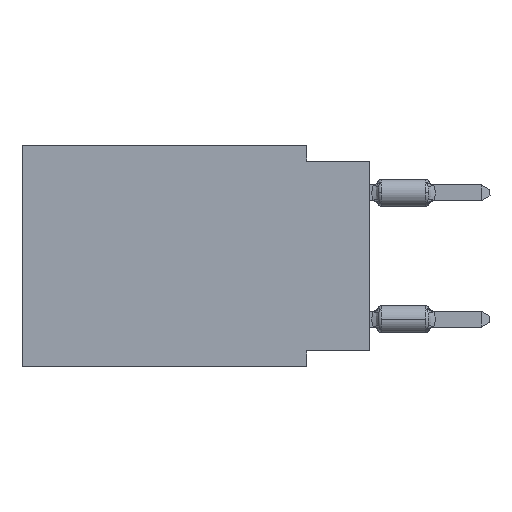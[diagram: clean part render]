
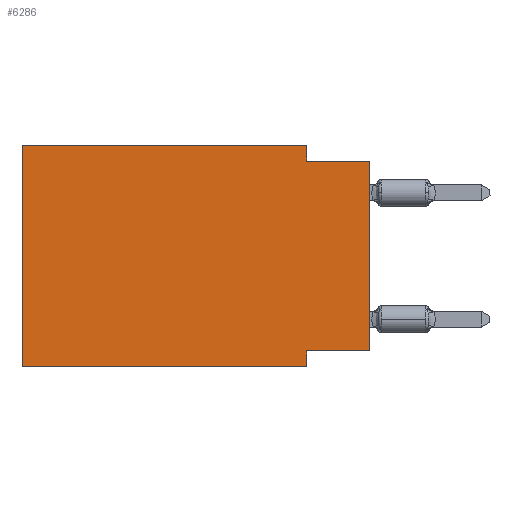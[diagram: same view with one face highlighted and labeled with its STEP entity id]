
A CAD part, left-side view. The second image highlights one B-rep face of the part: STEP entity #6286.
In plain terms, the highlighted planar face has unit normal (-1, 0, 0).
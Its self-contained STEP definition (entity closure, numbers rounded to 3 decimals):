
#235 = CARTESIAN_POINT ( 'NONE',  ( 0., 13.97, 0. ) ) ;
#1528 = LINE ( 'NONE', #235, #7803 ) ;
#1599 = ORIENTED_EDGE ( 'NONE', *, *, #19252, .T. ) ;
#1711 = ORIENTED_EDGE ( 'NONE', *, *, #14318, .F. ) ;
#1934 = LINE ( 'NONE', #18508, #4574 ) ;
#2109 = EDGE_CURVE ( 'NONE', #11399, #4119, #1528, .T. ) ;
#2158 = FACE_OUTER_BOUND ( 'NONE', #12468, .T. ) ;
#2733 = CARTESIAN_POINT ( 'NONE',  ( 0., 0., -8.255 ) ) ;
#2860 = ORIENTED_EDGE ( 'NONE', *, *, #2109, .F. ) ;
#3261 = ORIENTED_EDGE ( 'NONE', *, *, #16424, .T. ) ;
#3285 = LINE ( 'NONE', #11922, #14751 ) ;
#3541 = ORIENTED_EDGE ( 'NONE', *, *, #10617, .F. ) ;
#3924 = PLANE ( 'NONE',  #15400 ) ;
#4119 = VERTEX_POINT ( 'NONE', #5169 ) ;
#4137 = CARTESIAN_POINT ( 'NONE',  ( 0., 2.54, -8.255 ) ) ;
#4265 = CARTESIAN_POINT ( 'NONE',  ( 0., 13.97, 0. ) ) ;
#4369 = DIRECTION ( 'NONE',  ( 0., -1., 0. ) ) ;
#4574 = VECTOR ( 'NONE', #9362, 1000. ) ;
#4610 = VECTOR ( 'NONE', #14741, 1000. ) ;
#4696 = VERTEX_POINT ( 'NONE', #4137 ) ;
#4712 = CARTESIAN_POINT ( 'NONE',  ( 0., 2.54, -8.89 ) ) ;
#5099 = ORIENTED_EDGE ( 'NONE', *, *, #5491, .F. ) ;
#5169 = CARTESIAN_POINT ( 'NONE',  ( 0., 2.54, 0. ) ) ;
#5491 = EDGE_CURVE ( 'NONE', #9707, #11399, #12026, .T. ) ;
#6286 = ADVANCED_FACE ( 'NONE', ( #2158 ), #3924, .F. ) ;
#6368 = EDGE_CURVE ( 'NONE', #16617, #4696, #19417, .T. ) ;
#7644 = DIRECTION ( 'NONE',  ( 0., 0., 1. ) ) ;
#7803 = VECTOR ( 'NONE', #16904, 1000. ) ;
#8208 = DIRECTION ( 'NONE',  ( 1., 0., 0. ) ) ;
#8296 = VERTEX_POINT ( 'NONE', #9876 ) ;
#8310 = DIRECTION ( 'NONE',  ( 0., 0., -1. ) ) ;
#8923 = CARTESIAN_POINT ( 'NONE',  ( 0., 13.97, 0. ) ) ;
#9032 = VECTOR ( 'NONE', #7644, 1000. ) ;
#9362 = DIRECTION ( 'NONE',  ( 0., 0., 1. ) ) ;
#9707 = VERTEX_POINT ( 'NONE', #14753 ) ;
#9876 = CARTESIAN_POINT ( 'NONE',  ( 0., 0., -0.635 ) ) ;
#10180 = CARTESIAN_POINT ( 'NONE',  ( 0., 2.54, -8.89 ) ) ;
#10616 = LINE ( 'NONE', #15194, #17745 ) ;
#10617 = EDGE_CURVE ( 'NONE', #4696, #14006, #16153, .T. ) ;
#11399 = VERTEX_POINT ( 'NONE', #4265 ) ;
#11434 = VERTEX_POINT ( 'NONE', #14998 ) ;
#11641 = LINE ( 'NONE', #19292, #18827 ) ;
#11922 = CARTESIAN_POINT ( 'NONE',  ( 0., 13.97, -8.89 ) ) ;
#12023 = ORIENTED_EDGE ( 'NONE', *, *, #6368, .F. ) ;
#12026 = LINE ( 'NONE', #8923, #9032 ) ;
#12468 = EDGE_LOOP ( 'NONE', ( #1599, #1711, #17828, #2860, #5099, #3261, #3541, #12023 ) ) ;
#14006 = VERTEX_POINT ( 'NONE', #4712 ) ;
#14318 = EDGE_CURVE ( 'NONE', #11434, #8296, #10616, .T. ) ;
#14741 = DIRECTION ( 'NONE',  ( 0., 1., 0. ) ) ;
#14751 = VECTOR ( 'NONE', #4369, 1000. ) ;
#14753 = CARTESIAN_POINT ( 'NONE',  ( 0., 13.97, -8.89 ) ) ;
#14998 = CARTESIAN_POINT ( 'NONE',  ( 0., 2.54, -0.635 ) ) ;
#15042 = CARTESIAN_POINT ( 'NONE',  ( 0., 0., -8.255 ) ) ;
#15194 = CARTESIAN_POINT ( 'NONE',  ( 0., 0., -0.635 ) ) ;
#15400 = AXIS2_PLACEMENT_3D ( 'NONE', #18829, #8208, #18941 ) ;
#16153 = LINE ( 'NONE', #10180, #17291 ) ;
#16424 = EDGE_CURVE ( 'NONE', #9707, #14006, #3285, .T. ) ;
#16617 = VERTEX_POINT ( 'NONE', #2733 ) ;
#16779 = DIRECTION ( 'NONE',  ( 0., -1., 0. ) ) ;
#16904 = DIRECTION ( 'NONE',  ( 0., -1., 0. ) ) ;
#17291 = VECTOR ( 'NONE', #8310, 1000. ) ;
#17745 = VECTOR ( 'NONE', #16779, 1000. ) ;
#17828 = ORIENTED_EDGE ( 'NONE', *, *, #18639, .F. ) ;
#17986 = DIRECTION ( 'NONE',  ( 0., 0., -1. ) ) ;
#18508 = CARTESIAN_POINT ( 'NONE',  ( 0., 0., 0. ) ) ;
#18639 = EDGE_CURVE ( 'NONE', #4119, #11434, #11641, .T. ) ;
#18827 = VECTOR ( 'NONE', #17986, 1000. ) ;
#18829 = CARTESIAN_POINT ( 'NONE',  ( 0., 13.97, 0. ) ) ;
#18941 = DIRECTION ( 'NONE',  ( 0., 0., -1. ) ) ;
#19252 = EDGE_CURVE ( 'NONE', #16617, #8296, #1934, .T. ) ;
#19292 = CARTESIAN_POINT ( 'NONE',  ( 0., 2.54, 0. ) ) ;
#19417 = LINE ( 'NONE', #15042, #4610 ) ;
